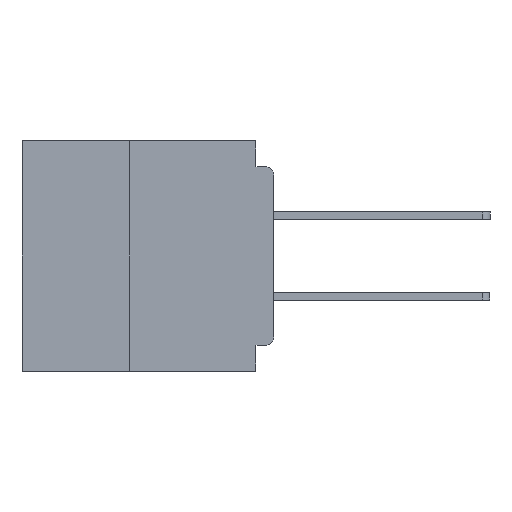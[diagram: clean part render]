
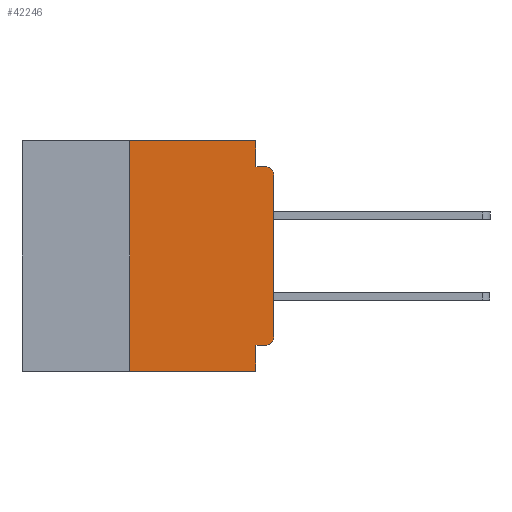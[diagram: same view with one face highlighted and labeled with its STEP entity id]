
A CAD part, left-side view. The second image highlights one B-rep face of the part: STEP entity #42246.
In plain terms, the highlighted planar face has unit normal (-1, 0, 0).
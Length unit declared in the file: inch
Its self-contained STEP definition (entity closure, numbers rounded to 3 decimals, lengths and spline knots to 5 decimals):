
#338 = VERTEX_POINT ( 'NONE', #31368 ) ;
#557 = VERTEX_POINT ( 'NONE', #6746 ) ;
#2121 = CARTESIAN_POINT ( 'NONE',  ( 0., 0., -0.045 ) ) ;
#2784 = EDGE_CURVE ( 'NONE', #34556, #557, #25712, .T. ) ;
#3039 = DIRECTION ( 'NONE',  ( 0., 0., -1. ) ) ;
#3086 = AXIS2_PLACEMENT_3D ( 'NONE', #39114, #19165, #42401 ) ;
#3740 = CARTESIAN_POINT ( 'NONE',  ( 0., 0., 0. ) ) ;
#3989 = ORIENTED_EDGE ( 'NONE', *, *, #29652, .T. ) ;
#4314 = VERTEX_POINT ( 'NONE', #23036 ) ;
#4644 = VECTOR ( 'NONE', #31580, 39.37008 ) ;
#4831 = LINE ( 'NONE', #11723, #10625 ) ;
#5710 = ORIENTED_EDGE ( 'NONE', *, *, #32492, .F. ) ;
#6389 = CARTESIAN_POINT ( 'NONE',  ( 0., 0.015, -0.06 ) ) ;
#6746 = CARTESIAN_POINT ( 'NONE',  ( 0., 0.25, 0. ) ) ;
#6902 = ORIENTED_EDGE ( 'NONE', *, *, #40183, .T. ) ;
#7129 = DIRECTION ( 'NONE',  ( 0., 0., 1. ) ) ;
#8911 = DIRECTION ( 'NONE',  ( 0., -1., 0. ) ) ;
#9265 = CARTESIAN_POINT ( 'NONE',  ( 0., 0.25, -0.4 ) ) ;
#9270 = DIRECTION ( 'NONE',  ( 0., -1., 0. ) ) ;
#9469 = CARTESIAN_POINT ( 'NONE',  ( 0., 0.031, -0.045 ) ) ;
#9760 = DIRECTION ( 'NONE',  ( 0., 0., -1. ) ) ;
#10625 = VECTOR ( 'NONE', #28511, 39.37008 ) ;
#10740 = CARTESIAN_POINT ( 'NONE',  ( 0., 0., -0.06 ) ) ;
#11723 = CARTESIAN_POINT ( 'NONE',  ( 0., 0., -0.355 ) ) ;
#12033 = ORIENTED_EDGE ( 'NONE', *, *, #14332, .T. ) ;
#12137 = FACE_OUTER_BOUND ( 'NONE', #23064, .T. ) ;
#12473 = LINE ( 'NONE', #3740, #30344 ) ;
#13357 = LINE ( 'NONE', #22610, #37932 ) ;
#13698 = EDGE_CURVE ( 'NONE', #338, #20125, #13357, .T. ) ;
#13748 = VERTEX_POINT ( 'NONE', #26299 ) ;
#13899 = ORIENTED_EDGE ( 'NONE', *, *, #2784, .F. ) ;
#14332 = EDGE_CURVE ( 'NONE', #26640, #33678, #31665, .T. ) ;
#14862 = EDGE_CURVE ( 'NONE', #26640, #13748, #4831, .T. ) ;
#15780 = PLANE ( 'NONE',  #22655 ) ;
#15928 = CARTESIAN_POINT ( 'NONE',  ( 0., 0.015, -0.355 ) ) ;
#16745 = VECTOR ( 'NONE', #42532, 39.37008 ) ;
#19165 = DIRECTION ( 'NONE',  ( -1., 0., 0. ) ) ;
#19586 = ORIENTED_EDGE ( 'NONE', *, *, #13698, .F. ) ;
#19828 = CARTESIAN_POINT ( 'NONE',  ( 0., 0.031, -0.4 ) ) ;
#20125 = VERTEX_POINT ( 'NONE', #9469 ) ;
#22258 = LINE ( 'NONE', #2121, #38879 ) ;
#22569 = DIRECTION ( 'NONE',  ( 0., 0., -1. ) ) ;
#22610 = CARTESIAN_POINT ( 'NONE',  ( 0., 0.031, 0. ) ) ;
#22655 = AXIS2_PLACEMENT_3D ( 'NONE', #39123, #42412, #22569 ) ;
#23036 = CARTESIAN_POINT ( 'NONE',  ( 0., 0.031, -0.4 ) ) ;
#23064 = EDGE_LOOP ( 'NONE', ( #28107, #6902, #37096, #19586, #31678, #13899, #3989, #5710, #27118, #12033 ) ) ;
#23625 = CARTESIAN_POINT ( 'NONE',  ( 0., 0., -0.34 ) ) ;
#24630 = EDGE_CURVE ( 'NONE', #557, #338, #30655, .T. ) ;
#25712 = LINE ( 'NONE', #9265, #16745 ) ;
#26009 = VECTOR ( 'NONE', #3039, 39.37008 ) ;
#26075 = CARTESIAN_POINT ( 'NONE',  ( 0., 0.437, 0. ) ) ;
#26299 = CARTESIAN_POINT ( 'NONE',  ( 0., 0.031, -0.355 ) ) ;
#26538 = CIRCLE ( 'NONE', #35130, 0.015 ) ;
#26640 = VERTEX_POINT ( 'NONE', #15928 ) ;
#27118 = ORIENTED_EDGE ( 'NONE', *, *, #14862, .F. ) ;
#28107 = ORIENTED_EDGE ( 'NONE', *, *, #38162, .T. ) ;
#28260 = CARTESIAN_POINT ( 'NONE',  ( 0., 0.437, -0.4 ) ) ;
#28511 = DIRECTION ( 'NONE',  ( 0., 1., 0. ) ) ;
#29652 = EDGE_CURVE ( 'NONE', #34556, #4314, #31434, .T. ) ;
#29885 = DIRECTION ( 'NONE',  ( -1., 0., 0. ) ) ;
#30344 = VECTOR ( 'NONE', #7129, 39.37008 ) ;
#30655 = LINE ( 'NONE', #26075, #38409 ) ;
#31368 = CARTESIAN_POINT ( 'NONE',  ( 0., 0.031, 0. ) ) ;
#31434 = LINE ( 'NONE', #28260, #4644 ) ;
#31580 = DIRECTION ( 'NONE',  ( 0., -1., 0. ) ) ;
#31640 = CARTESIAN_POINT ( 'NONE',  ( 0., 0.015, -0.045 ) ) ;
#31665 = CIRCLE ( 'NONE', #3086, 0.015 ) ;
#31678 = ORIENTED_EDGE ( 'NONE', *, *, #24630, .F. ) ;
#32492 = EDGE_CURVE ( 'NONE', #13748, #4314, #34806, .T. ) ;
#32642 = DIRECTION ( 'NONE',  ( 0., 0., -1. ) ) ;
#32816 = VERTEX_POINT ( 'NONE', #31640 ) ;
#33678 = VERTEX_POINT ( 'NONE', #23625 ) ;
#34556 = VERTEX_POINT ( 'NONE', #37785 ) ;
#34806 = LINE ( 'NONE', #19828, #26009 ) ;
#35130 = AXIS2_PLACEMENT_3D ( 'NONE', #6389, #29885, #9760 ) ;
#35305 = EDGE_CURVE ( 'NONE', #20125, #32816, #22258, .T. ) ;
#37096 = ORIENTED_EDGE ( 'NONE', *, *, #35305, .F. ) ;
#37785 = CARTESIAN_POINT ( 'NONE',  ( 0., 0.25, -0.4 ) ) ;
#37932 = VECTOR ( 'NONE', #32642, 39.37008 ) ;
#38162 = EDGE_CURVE ( 'NONE', #33678, #42551, #12473, .T. ) ;
#38409 = VECTOR ( 'NONE', #9270, 39.37008 ) ;
#38879 = VECTOR ( 'NONE', #8911, 39.37008 ) ;
#39114 = CARTESIAN_POINT ( 'NONE',  ( 0., 0.015, -0.34 ) ) ;
#39123 = CARTESIAN_POINT ( 'NONE',  ( 0., 0.437, 0. ) ) ;
#40183 = EDGE_CURVE ( 'NONE', #42551, #32816, #26538, .T. ) ;
#42246 = ADVANCED_FACE ( 'NONE', ( #12137 ), #15780, .F. ) ;
#42401 = DIRECTION ( 'NONE',  ( 0., 0., -1. ) ) ;
#42412 = DIRECTION ( 'NONE',  ( 1., 0., 0. ) ) ;
#42532 = DIRECTION ( 'NONE',  ( 0., 0., 1. ) ) ;
#42551 = VERTEX_POINT ( 'NONE', #10740 ) ;
